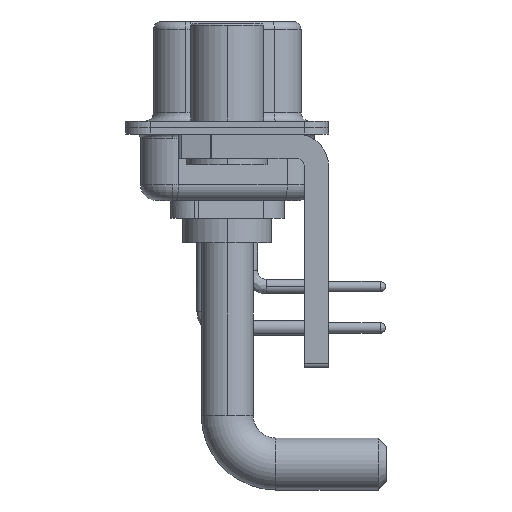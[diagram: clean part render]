
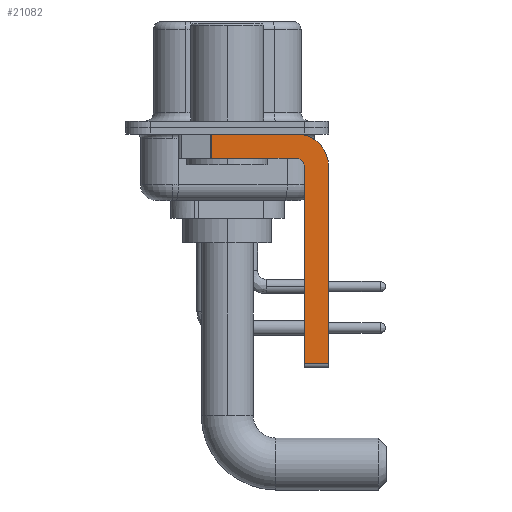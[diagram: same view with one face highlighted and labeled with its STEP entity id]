
A CAD part, left-side view. The second image highlights one B-rep face of the part: STEP entity #21082.
In plain terms, the highlighted planar face has unit normal (-1, 0, 0).
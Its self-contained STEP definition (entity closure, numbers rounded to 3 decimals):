
#231 = DIRECTION ( 'NONE',  ( -1., 0., 0. ) ) ;
#266 = AXIS2_PLACEMENT_3D ( 'NONE', #4492, #231, #10495 ) ;
#467 = CIRCLE ( 'NONE', #3656, 2. ) ;
#980 = DIRECTION ( 'NONE',  ( 1., 0., 0. ) ) ;
#1280 = DIRECTION ( 'NONE',  ( 0., 0., -1. ) ) ;
#1969 = EDGE_CURVE ( 'NONE', #12134, #22461, #25947, .T. ) ;
#2761 = LINE ( 'NONE', #15717, #18758 ) ;
#2960 = DIRECTION ( 'NONE',  ( 0., 0., -1. ) ) ;
#3401 = PLANE ( 'NONE',  #4968 ) ;
#3576 = DIRECTION ( 'NONE',  ( 0., 0., -1. ) ) ;
#3656 = AXIS2_PLACEMENT_3D ( 'NONE', #16214, #980, #2960 ) ;
#3686 = CARTESIAN_POINT ( 'NONE',  ( -2.9, -4.25, -2.4 ) ) ;
#4140 = EDGE_CURVE ( 'NONE', #13490, #17612, #21172, .T. ) ;
#4492 = CARTESIAN_POINT ( 'NONE',  ( -2.9, -4.25, -2.4 ) ) ;
#4551 = EDGE_CURVE ( 'NONE', #12134, #14391, #27983, .T. ) ;
#4799 = VERTEX_POINT ( 'NONE', #26255 ) ;
#4861 = VECTOR ( 'NONE', #9657, 1000. ) ;
#4958 = CARTESIAN_POINT ( 'NONE',  ( -2.9, -4.25, -1.9 ) ) ;
#4968 = AXIS2_PLACEMENT_3D ( 'NONE', #3686, #9815, #1280 ) ;
#5241 = LINE ( 'NONE', #4958, #4861 ) ;
#5752 = EDGE_CURVE ( 'NONE', #14391, #6588, #467, .T. ) ;
#5805 = ORIENTED_EDGE ( 'NONE', *, *, #15936, .F. ) ;
#6043 = EDGE_CURVE ( 'NONE', #6581, #13490, #2761, .T. ) ;
#6581 = VERTEX_POINT ( 'NONE', #17340 ) ;
#6588 = VERTEX_POINT ( 'NONE', #27902 ) ;
#9229 = ORIENTED_EDGE ( 'NONE', *, *, #4551, .F. ) ;
#9657 = DIRECTION ( 'NONE',  ( 0., 1., 0. ) ) ;
#9815 = DIRECTION ( 'NONE',  ( 1., 0., 0. ) ) ;
#9991 = CARTESIAN_POINT ( 'NONE',  ( -2.9, -6.25, -2.4 ) ) ;
#10113 = CARTESIAN_POINT ( 'NONE',  ( -2.9, 0.978, -1.9 ) ) ;
#10495 = DIRECTION ( 'NONE',  ( 0., 0., 1. ) ) ;
#10774 = ORIENTED_EDGE ( 'NONE', *, *, #19269, .F. ) ;
#11166 = DIRECTION ( 'NONE',  ( 0., 0., 1. ) ) ;
#11625 = CARTESIAN_POINT ( 'NONE',  ( -2.9, -4.25, -1.9 ) ) ;
#11949 = FACE_OUTER_BOUND ( 'NONE', #18811, .T. ) ;
#12134 = VERTEX_POINT ( 'NONE', #19309 ) ;
#12215 = DIRECTION ( 'NONE',  ( 0., 0., -1. ) ) ;
#13490 = VERTEX_POINT ( 'NONE', #24584 ) ;
#13511 = DIRECTION ( 'NONE',  ( 0., -1., 0. ) ) ;
#13650 = VECTOR ( 'NONE', #23542, 1000. ) ;
#13771 = ORIENTED_EDGE ( 'NONE', *, *, #17090, .T. ) ;
#13979 = LINE ( 'NONE', #9991, #26253 ) ;
#14391 = VERTEX_POINT ( 'NONE', #20089 ) ;
#15717 = CARTESIAN_POINT ( 'NONE',  ( -2.9, -4.75, -14.8 ) ) ;
#15936 = EDGE_CURVE ( 'NONE', #17612, #22461, #5241, .T. ) ;
#16214 = CARTESIAN_POINT ( 'NONE',  ( -2.9, -4.25, -2.4 ) ) ;
#16731 = ORIENTED_EDGE ( 'NONE', *, *, #5752, .F. ) ;
#17090 = EDGE_CURVE ( 'NONE', #6581, #4799, #24325, .T. ) ;
#17340 = CARTESIAN_POINT ( 'NONE',  ( -2.9, -4.75, -14.55 ) ) ;
#17355 = CARTESIAN_POINT ( 'NONE',  ( -2.9, -4.25, -14.55 ) ) ;
#17612 = VERTEX_POINT ( 'NONE', #11625 ) ;
#18461 = CARTESIAN_POINT ( 'NONE',  ( -2.9, 0.978, -1.9 ) ) ;
#18758 = VECTOR ( 'NONE', #11166, 1000. ) ;
#18811 = EDGE_LOOP ( 'NONE', ( #9229, #20566, #5805, #20989, #23729, #13771, #10774, #16731 ) ) ;
#19269 = EDGE_CURVE ( 'NONE', #6588, #4799, #13979, .T. ) ;
#19309 = CARTESIAN_POINT ( 'NONE',  ( -2.9, 0.978, -0.4 ) ) ;
#20089 = CARTESIAN_POINT ( 'NONE',  ( -2.9, -4.25, -0.4 ) ) ;
#20566 = ORIENTED_EDGE ( 'NONE', *, *, #1969, .T. ) ;
#20989 = ORIENTED_EDGE ( 'NONE', *, *, #4140, .F. ) ;
#21082 = ADVANCED_FACE ( 'NONE', ( #11949 ), #3401, .F. ) ;
#21172 = CIRCLE ( 'NONE', #266, 0.5 ) ;
#22023 = VECTOR ( 'NONE', #12215, 1000. ) ;
#22461 = VERTEX_POINT ( 'NONE', #10113 ) ;
#23542 = DIRECTION ( 'NONE',  ( 0., -1., 0. ) ) ;
#23729 = ORIENTED_EDGE ( 'NONE', *, *, #6043, .F. ) ;
#24325 = LINE ( 'NONE', #17355, #24863 ) ;
#24584 = CARTESIAN_POINT ( 'NONE',  ( -2.9, -4.75, -2.4 ) ) ;
#24863 = VECTOR ( 'NONE', #13511, 1000. ) ;
#25947 = LINE ( 'NONE', #18461, #22023 ) ;
#26253 = VECTOR ( 'NONE', #3576, 1000. ) ;
#26255 = CARTESIAN_POINT ( 'NONE',  ( -2.9, -6.25, -14.55 ) ) ;
#27705 = CARTESIAN_POINT ( 'NONE',  ( -2.9, 3., -0.4 ) ) ;
#27902 = CARTESIAN_POINT ( 'NONE',  ( -2.9, -6.25, -2.4 ) ) ;
#27983 = LINE ( 'NONE', #27705, #13650 ) ;
